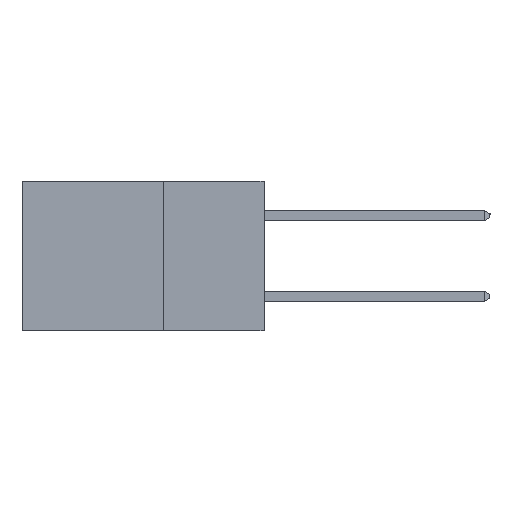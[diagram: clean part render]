
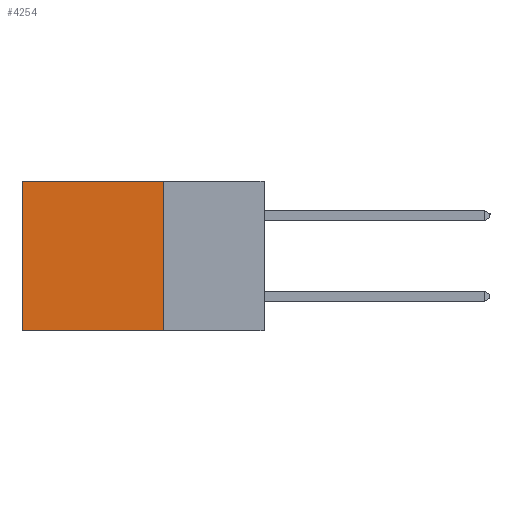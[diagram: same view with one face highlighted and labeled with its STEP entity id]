
A CAD part, left-side view. The second image highlights one B-rep face of the part: STEP entity #4254.
In plain terms, the highlighted planar face has unit normal (-1, 0, 0).
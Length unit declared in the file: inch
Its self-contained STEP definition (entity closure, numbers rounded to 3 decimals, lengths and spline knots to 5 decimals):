
#29 = VECTOR ( 'NONE', #4047, 39.37008 ) ;
#131 = CARTESIAN_POINT ( 'NONE',  ( 0.298, 0.6, 0. ) ) ;
#196 = ORIENTED_EDGE ( 'NONE', *, *, #4161, .T. ) ;
#264 = DIRECTION ( 'NONE',  ( 1., 0., 0. ) ) ;
#390 = LINE ( 'NONE', #131, #29 ) ;
#455 = CARTESIAN_POINT ( 'NONE',  ( 0.298, 0.25, 0. ) ) ;
#497 = ORIENTED_EDGE ( 'NONE', *, *, #3957, .F. ) ;
#584 = ORIENTED_EDGE ( 'NONE', *, *, #6131, .T. ) ;
#597 = CARTESIAN_POINT ( 'NONE',  ( 0.298, 0.25, -0.37 ) ) ;
#1057 = CARTESIAN_POINT ( 'NONE',  ( 0.298, 0.6, -0.37 ) ) ;
#1213 = CARTESIAN_POINT ( 'NONE',  ( 0.298, 0.25, 0. ) ) ;
#1979 = ORIENTED_EDGE ( 'NONE', *, *, #9029, .F. ) ;
#2117 = DIRECTION ( 'NONE',  ( 0., 1., 0. ) ) ;
#3315 = VERTEX_POINT ( 'NONE', #7086 ) ;
#3957 = EDGE_CURVE ( 'NONE', #3315, #8323, #11952, .T. ) ;
#4047 = DIRECTION ( 'NONE',  ( 0., 0., -1. ) ) ;
#4095 = VECTOR ( 'NONE', #6140, 39.37008 ) ;
#4161 = EDGE_CURVE ( 'NONE', #8115, #11815, #390, .T. ) ;
#4254 = ADVANCED_FACE ( 'NONE', ( #10087 ), #10988, .F. ) ;
#5680 = VECTOR ( 'NONE', #9782, 39.37008 ) ;
#6131 = EDGE_CURVE ( 'NONE', #3315, #8115, #8691, .T. ) ;
#6140 = DIRECTION ( 'NONE',  ( 0., 0., -1. ) ) ;
#6276 = CARTESIAN_POINT ( 'NONE',  ( 0.298, 0.25, 0. ) ) ;
#7086 = CARTESIAN_POINT ( 'NONE',  ( 0.298, 0.25, 0. ) ) ;
#7779 = DIRECTION ( 'NONE',  ( 0., 0., -1. ) ) ;
#8097 = AXIS2_PLACEMENT_3D ( 'NONE', #1213, #264, #7779 ) ;
#8115 = VERTEX_POINT ( 'NONE', #12021 ) ;
#8323 = VERTEX_POINT ( 'NONE', #597 ) ;
#8691 = LINE ( 'NONE', #455, #5680 ) ;
#9029 = EDGE_CURVE ( 'NONE', #8323, #11815, #11063, .T. ) ;
#9474 = VECTOR ( 'NONE', #2117, 39.37008 ) ;
#9782 = DIRECTION ( 'NONE',  ( 0., 1., 0. ) ) ;
#10087 = FACE_OUTER_BOUND ( 'NONE', #10677, .T. ) ;
#10434 = CARTESIAN_POINT ( 'NONE',  ( 0.298, 0.25, -0.37 ) ) ;
#10677 = EDGE_LOOP ( 'NONE', ( #196, #1979, #497, #584 ) ) ;
#10988 = PLANE ( 'NONE',  #8097 ) ;
#11063 = LINE ( 'NONE', #10434, #9474 ) ;
#11815 = VERTEX_POINT ( 'NONE', #1057 ) ;
#11952 = LINE ( 'NONE', #6276, #4095 ) ;
#12021 = CARTESIAN_POINT ( 'NONE',  ( 0.298, 0.6, 0. ) ) ;
